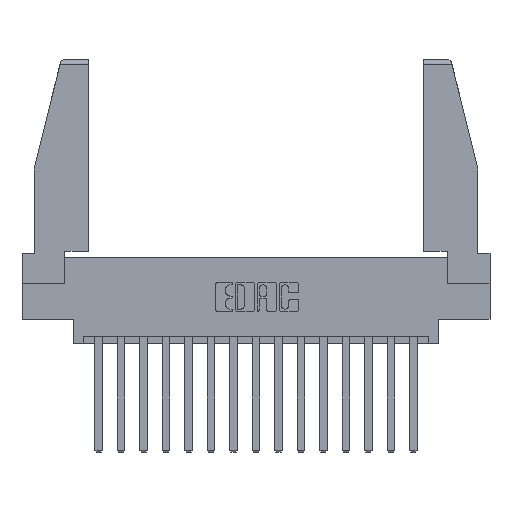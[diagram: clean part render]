
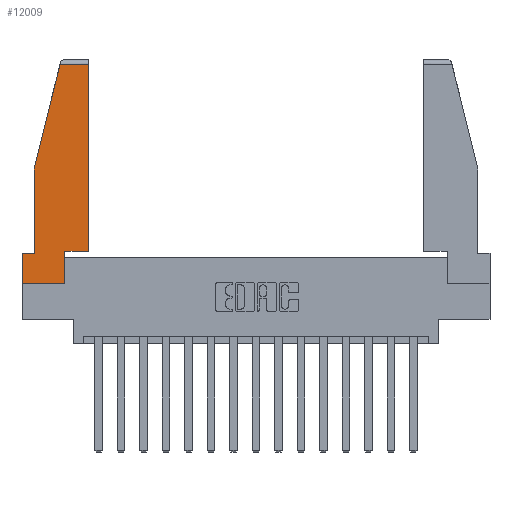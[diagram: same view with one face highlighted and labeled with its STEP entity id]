
A CAD part, top view. The second image highlights one B-rep face of the part: STEP entity #12009.
In plain terms, the highlighted planar face has unit normal (0, 0, 1).
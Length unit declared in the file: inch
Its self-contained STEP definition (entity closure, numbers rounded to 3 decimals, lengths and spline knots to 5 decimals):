
#172 = CARTESIAN_POINT ( 'NONE',  ( 0., 0.21, 0. ) ) ;
#426 = CARTESIAN_POINT ( 'NONE',  ( 0.461, 0.223, 0. ) ) ;
#1017 = VERTEX_POINT ( 'NONE', #11976 ) ;
#1220 = CARTESIAN_POINT ( 'NONE',  ( 0.297, 0., 0. ) ) ;
#1317 = EDGE_CURVE ( 'NONE', #16110, #2366, #14279, .T. ) ;
#1437 = ORIENTED_EDGE ( 'NONE', *, *, #11663, .T. ) ;
#2366 = VERTEX_POINT ( 'NONE', #16147 ) ;
#2390 = PLANE ( 'NONE',  #12250 ) ;
#2814 = DIRECTION ( 'NONE',  ( 0., 1., 0. ) ) ;
#2904 = CARTESIAN_POINT ( 'NONE',  ( 0., 0.21, 0. ) ) ;
#3018 = CARTESIAN_POINT ( 'NONE',  ( 0.461, 0.223, 0. ) ) ;
#3130 = DIRECTION ( 'NONE',  ( 0., 1., 0. ) ) ;
#3239 = FACE_OUTER_BOUND ( 'NONE', #13564, .T. ) ;
#3581 = LINE ( 'NONE', #2904, #9936 ) ;
#4105 = VERTEX_POINT ( 'NONE', #9528 ) ;
#4150 = CARTESIAN_POINT ( 'NONE',  ( 0.271, 1.55, 0. ) ) ;
#4450 = EDGE_CURVE ( 'NONE', #13300, #4567, #12357, .T. ) ;
#4567 = VERTEX_POINT ( 'NONE', #9587 ) ;
#4629 = LINE ( 'NONE', #3018, #5905 ) ;
#4732 = ORIENTED_EDGE ( 'NONE', *, *, #6852, .T. ) ;
#5478 = LINE ( 'NONE', #16229, #16901 ) ;
#5905 = VECTOR ( 'NONE', #3130, 39.37008 ) ;
#6302 = CARTESIAN_POINT ( 'NONE',  ( 0., 0., 0. ) ) ;
#6362 = LINE ( 'NONE', #11947, #7658 ) ;
#6464 = LINE ( 'NONE', #10368, #10265 ) ;
#6607 = VERTEX_POINT ( 'NONE', #426 ) ;
#6685 = DIRECTION ( 'NONE',  ( 1., 0., 0. ) ) ;
#6852 = EDGE_CURVE ( 'NONE', #15687, #17223, #6362, .T. ) ;
#7051 = ORIENTED_EDGE ( 'NONE', *, *, #16557, .T. ) ;
#7228 = ORIENTED_EDGE ( 'NONE', *, *, #4450, .T. ) ;
#7658 = VECTOR ( 'NONE', #6685, 39.37008 ) ;
#7809 = ORIENTED_EDGE ( 'NONE', *, *, #1317, .T. ) ;
#7857 = EDGE_CURVE ( 'NONE', #4105, #13300, #5478, .T. ) ;
#8034 = CARTESIAN_POINT ( 'NONE',  ( 0.086, 0.21, 0. ) ) ;
#9493 = DIRECTION ( 'NONE',  ( -1., 0., 0. ) ) ;
#9528 = CARTESIAN_POINT ( 'NONE',  ( 0.461, 1.52, 0. ) ) ;
#9587 = CARTESIAN_POINT ( 'NONE',  ( 0.086, 0.8, 0. ) ) ;
#9651 = DIRECTION ( 'NONE',  ( -1., 0., 0. ) ) ;
#9840 = EDGE_CURVE ( 'NONE', #6607, #4105, #4629, .T. ) ;
#9936 = VECTOR ( 'NONE', #16453, 39.37008 ) ;
#10265 = VECTOR ( 'NONE', #14900, 39.37008 ) ;
#10368 = CARTESIAN_POINT ( 'NONE',  ( 0.297, 0.223, 0. ) ) ;
#10668 = VECTOR ( 'NONE', #9651, 39.37008 ) ;
#11059 = ORIENTED_EDGE ( 'NONE', *, *, #7857, .T. ) ;
#11301 = ORIENTED_EDGE ( 'NONE', *, *, #9840, .T. ) ;
#11319 = VECTOR ( 'NONE', #13852, 39.37008 ) ;
#11663 = EDGE_CURVE ( 'NONE', #17223, #1017, #13998, .T. ) ;
#11812 = DIRECTION ( 'NONE',  ( 0., 0., 1. ) ) ;
#11919 = CARTESIAN_POINT ( 'NONE',  ( 0., 0., 0. ) ) ;
#11947 = CARTESIAN_POINT ( 'NONE',  ( 0., 0., 0. ) ) ;
#11976 = CARTESIAN_POINT ( 'NONE',  ( 0.297, 0.223, 0. ) ) ;
#12009 = ADVANCED_FACE ( 'NONE', ( #3239 ), #2390, .T. ) ;
#12250 = AXIS2_PLACEMENT_3D ( 'NONE', #11919, #11812, #15903 ) ;
#12357 = LINE ( 'NONE', #4150, #13894 ) ;
#12448 = CARTESIAN_POINT ( 'NONE',  ( 0.086, 0.8, 0. ) ) ;
#12764 = LINE ( 'NONE', #12448, #11319 ) ;
#13300 = VERTEX_POINT ( 'NONE', #15328 ) ;
#13330 = DIRECTION ( 'NONE',  ( -0.239, -0.971, 0. ) ) ;
#13564 = EDGE_LOOP ( 'NONE', ( #11301, #11059, #7228, #17517, #7809, #16891, #4732, #1437, #7051 ) ) ;
#13760 = CARTESIAN_POINT ( 'NONE',  ( 0.297, 0., 0. ) ) ;
#13852 = DIRECTION ( 'NONE',  ( 0., -1., 0. ) ) ;
#13894 = VECTOR ( 'NONE', #13330, 39.37008 ) ;
#13998 = LINE ( 'NONE', #13760, #14815 ) ;
#14279 = LINE ( 'NONE', #172, #10668 ) ;
#14700 = EDGE_CURVE ( 'NONE', #2366, #15687, #3581, .T. ) ;
#14815 = VECTOR ( 'NONE', #2814, 39.37008 ) ;
#14900 = DIRECTION ( 'NONE',  ( 1., 0., 0. ) ) ;
#15328 = CARTESIAN_POINT ( 'NONE',  ( 0.2636, 1.52, 0. ) ) ;
#15687 = VERTEX_POINT ( 'NONE', #6302 ) ;
#15903 = DIRECTION ( 'NONE',  ( 1., 0., 0. ) ) ;
#16110 = VERTEX_POINT ( 'NONE', #8034 ) ;
#16147 = CARTESIAN_POINT ( 'NONE',  ( 0., 0.21, 0. ) ) ;
#16229 = CARTESIAN_POINT ( 'NONE',  ( 0., 1.52, 0. ) ) ;
#16453 = DIRECTION ( 'NONE',  ( 0., -1., 0. ) ) ;
#16557 = EDGE_CURVE ( 'NONE', #1017, #6607, #6464, .T. ) ;
#16891 = ORIENTED_EDGE ( 'NONE', *, *, #14700, .T. ) ;
#16901 = VECTOR ( 'NONE', #9493, 39.37008 ) ;
#16961 = EDGE_CURVE ( 'NONE', #4567, #16110, #12764, .T. ) ;
#17223 = VERTEX_POINT ( 'NONE', #1220 ) ;
#17517 = ORIENTED_EDGE ( 'NONE', *, *, #16961, .T. ) ;
